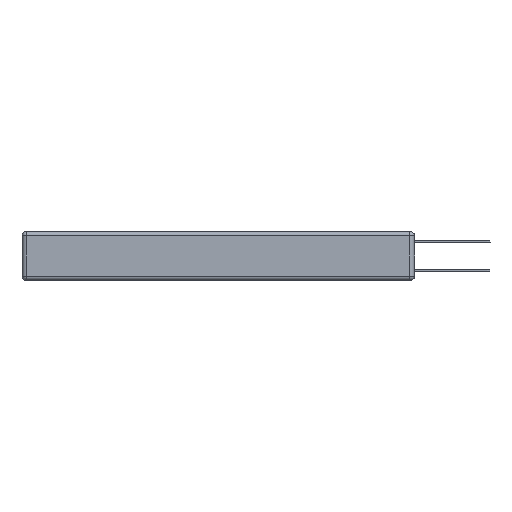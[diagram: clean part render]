
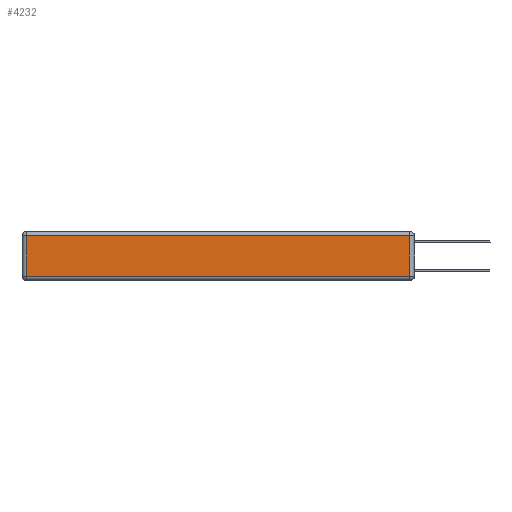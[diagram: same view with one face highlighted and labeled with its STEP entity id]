
A CAD part, left-side view. The second image highlights one B-rep face of the part: STEP entity #4232.
In plain terms, the highlighted planar face has unit normal (-1, 0, 0).
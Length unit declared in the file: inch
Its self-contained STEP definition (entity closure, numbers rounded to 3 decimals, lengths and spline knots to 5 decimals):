
#116 = VERTEX_POINT ( 'NONE', #11088 ) ;
#1234 = DIRECTION ( 'NONE',  ( 0., -1., 0. ) ) ;
#1343 = EDGE_CURVE ( 'NONE', #116, #5975, #11249, .T. ) ;
#1423 = EDGE_LOOP ( 'NONE', ( #1472, #7504, #7399, #5303 ) ) ;
#1472 = ORIENTED_EDGE ( 'NONE', *, *, #8132, .T. ) ;
#1535 = FACE_OUTER_BOUND ( 'NONE', #1423, .T. ) ;
#1631 = VECTOR ( 'NONE', #1234, 39.37008 ) ;
#1756 = DIRECTION ( 'NONE',  ( 0., 0., -1. ) ) ;
#2011 = VECTOR ( 'NONE', #7664, 39.37008 ) ;
#2099 = DIRECTION ( 'NONE',  ( -1., 0., 0. ) ) ;
#2751 = CARTESIAN_POINT ( 'NONE',  ( 0., 0.03, -0.343 ) ) ;
#2972 = EDGE_CURVE ( 'NONE', #5975, #4794, #4573, .T. ) ;
#3177 = CARTESIAN_POINT ( 'NONE',  ( 0., 2.72, -0.313 ) ) ;
#4232 = ADVANCED_FACE ( 'NONE', ( #1535 ), #4969, .T. ) ;
#4573 = LINE ( 'NONE', #9627, #2011 ) ;
#4794 = VERTEX_POINT ( 'NONE', #11613 ) ;
#4796 = CARTESIAN_POINT ( 'NONE',  ( 0., 0.03, -0.03 ) ) ;
#4881 = CARTESIAN_POINT ( 'NONE',  ( 0., 0., -0.343 ) ) ;
#4969 = PLANE ( 'NONE',  #12114 ) ;
#5303 = ORIENTED_EDGE ( 'NONE', *, *, #7103, .T. ) ;
#5558 = LINE ( 'NONE', #11980, #1631 ) ;
#5975 = VERTEX_POINT ( 'NONE', #4796 ) ;
#7103 = EDGE_CURVE ( 'NONE', #4794, #9182, #9249, .T. ) ;
#7399 = ORIENTED_EDGE ( 'NONE', *, *, #2972, .T. ) ;
#7504 = ORIENTED_EDGE ( 'NONE', *, *, #1343, .T. ) ;
#7616 = VECTOR ( 'NONE', #12473, 39.37008 ) ;
#7664 = DIRECTION ( 'NONE',  ( 0., 1., 0. ) ) ;
#8132 = EDGE_CURVE ( 'NONE', #9182, #116, #5558, .T. ) ;
#9182 = VERTEX_POINT ( 'NONE', #3177 ) ;
#9249 = LINE ( 'NONE', #12427, #10272 ) ;
#9627 = CARTESIAN_POINT ( 'NONE',  ( 0., 2.75, -0.03 ) ) ;
#10272 = VECTOR ( 'NONE', #1756, 39.37008 ) ;
#10625 = DIRECTION ( 'NONE',  ( 0., 0., 1. ) ) ;
#11088 = CARTESIAN_POINT ( 'NONE',  ( 0., 0.03, -0.313 ) ) ;
#11249 = LINE ( 'NONE', #2751, #7616 ) ;
#11613 = CARTESIAN_POINT ( 'NONE',  ( 0., 2.72, -0.03 ) ) ;
#11980 = CARTESIAN_POINT ( 'NONE',  ( 0., 0., -0.313 ) ) ;
#12114 = AXIS2_PLACEMENT_3D ( 'NONE', #4881, #2099, #10625 ) ;
#12427 = CARTESIAN_POINT ( 'NONE',  ( 0., 2.72, -0.343 ) ) ;
#12473 = DIRECTION ( 'NONE',  ( 0., 0., 1. ) ) ;
